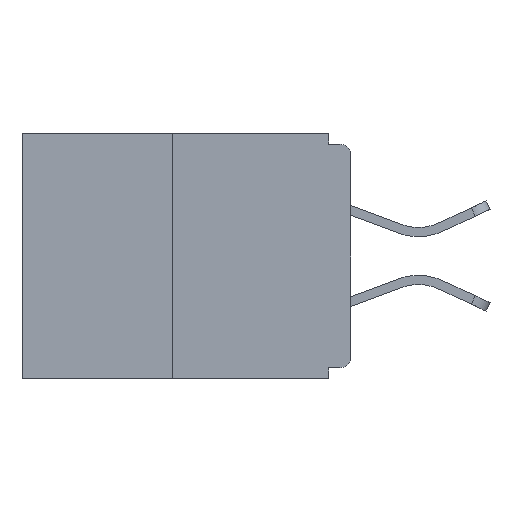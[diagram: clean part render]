
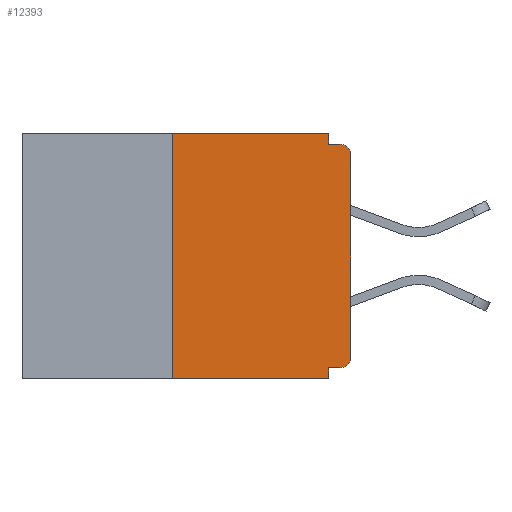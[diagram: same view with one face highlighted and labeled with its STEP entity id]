
A CAD part, left-side view. The second image highlights one B-rep face of the part: STEP entity #12393.
In plain terms, the highlighted planar face has unit normal (-1, 0, 0).
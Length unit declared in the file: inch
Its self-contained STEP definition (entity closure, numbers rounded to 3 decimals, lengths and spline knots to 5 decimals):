
#35 = ORIENTED_EDGE ( 'NONE', *, *, #10973, .T. ) ;
#58 = CARTESIAN_POINT ( 'NONE',  ( 0., 0., -0.03 ) ) ;
#764 = DIRECTION ( 'NONE',  ( 0., 0., -1. ) ) ;
#807 = VECTOR ( 'NONE', #6528, 39.37008 ) ;
#816 = EDGE_CURVE ( 'NONE', #4994, #9443, #3409, .T. ) ;
#1042 = DIRECTION ( 'NONE',  ( 0., 0., -1. ) ) ;
#1137 = CARTESIAN_POINT ( 'NONE',  ( 0., 0.031, -0.328 ) ) ;
#1309 = ORIENTED_EDGE ( 'NONE', *, *, #11805, .F. ) ;
#1310 = ORIENTED_EDGE ( 'NONE', *, *, #8022, .F. ) ;
#1621 = ORIENTED_EDGE ( 'NONE', *, *, #11924, .F. ) ;
#1691 = VERTEX_POINT ( 'NONE', #15045 ) ;
#1877 = ORIENTED_EDGE ( 'NONE', *, *, #17465, .F. ) ;
#2968 = CARTESIAN_POINT ( 'NONE',  ( 0., 0.46, -0.343 ) ) ;
#2973 = EDGE_CURVE ( 'NONE', #4994, #1691, #9009, .T. ) ;
#2989 = ORIENTED_EDGE ( 'NONE', *, *, #15163, .T. ) ;
#3265 = DIRECTION ( 'NONE',  ( 0., -1., 0. ) ) ;
#3409 = LINE ( 'NONE', #2968, #13923 ) ;
#3988 = DIRECTION ( 'NONE',  ( 0., -1., 0. ) ) ;
#4111 = CARTESIAN_POINT ( 'NONE',  ( 0., 0.46, 0. ) ) ;
#4182 = DIRECTION ( 'NONE',  ( 0., 0., -1. ) ) ;
#4279 = VERTEX_POINT ( 'NONE', #58 ) ;
#4339 = CARTESIAN_POINT ( 'NONE',  ( 0., 0., -0.015 ) ) ;
#4845 = ORIENTED_EDGE ( 'NONE', *, *, #12919, .F. ) ;
#4859 = CARTESIAN_POINT ( 'NONE',  ( 0., 0.015, -0.313 ) ) ;
#4976 = CARTESIAN_POINT ( 'NONE',  ( 0., 0.015, -0.015 ) ) ;
#4994 = VERTEX_POINT ( 'NONE', #15820 ) ;
#5221 = CARTESIAN_POINT ( 'NONE',  ( 0., 0.46, 0. ) ) ;
#5409 = CARTESIAN_POINT ( 'NONE',  ( 0., 0.031, -0.343 ) ) ;
#5436 = CIRCLE ( 'NONE', #13734, 0.015 ) ;
#5612 = CARTESIAN_POINT ( 'NONE',  ( 0., 0.015, -0.03 ) ) ;
#5796 = VERTEX_POINT ( 'NONE', #10168 ) ;
#6383 = LINE ( 'NONE', #7894, #13456 ) ;
#6528 = DIRECTION ( 'NONE',  ( 0., 0., 1. ) ) ;
#6610 = DIRECTION ( 'NONE',  ( 0., 0., -1. ) ) ;
#7894 = CARTESIAN_POINT ( 'NONE',  ( 0., 0.031, 0. ) ) ;
#8022 = EDGE_CURVE ( 'NONE', #14456, #11854, #15405, .T. ) ;
#8230 = DIRECTION ( 'NONE',  ( 0., 0., 1. ) ) ;
#8938 = DIRECTION ( 'NONE',  ( -1., 0., 0. ) ) ;
#9009 = LINE ( 'NONE', #9546, #14568 ) ;
#9185 = VECTOR ( 'NONE', #3265, 39.37008 ) ;
#9206 = CARTESIAN_POINT ( 'NONE',  ( 0., 0., -0.328 ) ) ;
#9443 = VERTEX_POINT ( 'NONE', #11286 ) ;
#9546 = CARTESIAN_POINT ( 'NONE',  ( 0., 0.25, 0. ) ) ;
#9635 = CIRCLE ( 'NONE', #11401, 0.015 ) ;
#9689 = LINE ( 'NONE', #4111, #10969 ) ;
#10168 = CARTESIAN_POINT ( 'NONE',  ( 0., 0., -0.313 ) ) ;
#10370 = CARTESIAN_POINT ( 'NONE',  ( 0., 0., 0. ) ) ;
#10440 = ORIENTED_EDGE ( 'NONE', *, *, #14248, .T. ) ;
#10583 = DIRECTION ( 'NONE',  ( 0., 1., 0. ) ) ;
#10796 = LINE ( 'NONE', #5409, #12995 ) ;
#10889 = ORIENTED_EDGE ( 'NONE', *, *, #816, .T. ) ;
#10969 = VECTOR ( 'NONE', #3988, 39.37008 ) ;
#10973 = EDGE_CURVE ( 'NONE', #4279, #11854, #5436, .T. ) ;
#11286 = CARTESIAN_POINT ( 'NONE',  ( 0., 0.031, -0.343 ) ) ;
#11401 = AXIS2_PLACEMENT_3D ( 'NONE', #4859, #8938, #764 ) ;
#11497 = VERTEX_POINT ( 'NONE', #14075 ) ;
#11805 = EDGE_CURVE ( 'NONE', #16619, #13224, #11896, .T. ) ;
#11854 = VERTEX_POINT ( 'NONE', #4976 ) ;
#11896 = LINE ( 'NONE', #9206, #16620 ) ;
#11924 = EDGE_CURVE ( 'NONE', #13224, #9443, #10796, .T. ) ;
#12102 = DIRECTION ( 'NONE',  ( 0., 0., -1. ) ) ;
#12197 = DIRECTION ( 'NONE',  ( 1., 0., 0. ) ) ;
#12393 = ADVANCED_FACE ( 'NONE', ( #14213 ), #17614, .F. ) ;
#12407 = LINE ( 'NONE', #10370, #807 ) ;
#12708 = ORIENTED_EDGE ( 'NONE', *, *, #2973, .F. ) ;
#12767 = DIRECTION ( 'NONE',  ( 0., -1., 0. ) ) ;
#12919 = EDGE_CURVE ( 'NONE', #1691, #11497, #9689, .T. ) ;
#12995 = VECTOR ( 'NONE', #12102, 39.37008 ) ;
#13099 = CARTESIAN_POINT ( 'NONE',  ( 0., 0.015, -0.328 ) ) ;
#13224 = VERTEX_POINT ( 'NONE', #1137 ) ;
#13456 = VECTOR ( 'NONE', #1042, 39.37008 ) ;
#13460 = AXIS2_PLACEMENT_3D ( 'NONE', #5221, #12197, #6610 ) ;
#13734 = AXIS2_PLACEMENT_3D ( 'NONE', #5612, #15278, #4182 ) ;
#13923 = VECTOR ( 'NONE', #12767, 39.37008 ) ;
#14075 = CARTESIAN_POINT ( 'NONE',  ( 0., 0.031, 0. ) ) ;
#14213 = FACE_OUTER_BOUND ( 'NONE', #17084, .T. ) ;
#14248 = EDGE_CURVE ( 'NONE', #16619, #5796, #9635, .T. ) ;
#14456 = VERTEX_POINT ( 'NONE', #16349 ) ;
#14568 = VECTOR ( 'NONE', #8230, 39.37008 ) ;
#15045 = CARTESIAN_POINT ( 'NONE',  ( 0., 0.25, 0. ) ) ;
#15163 = EDGE_CURVE ( 'NONE', #5796, #4279, #12407, .T. ) ;
#15278 = DIRECTION ( 'NONE',  ( -1., 0., 0. ) ) ;
#15405 = LINE ( 'NONE', #4339, #9185 ) ;
#15820 = CARTESIAN_POINT ( 'NONE',  ( 0., 0.25, -0.343 ) ) ;
#16349 = CARTESIAN_POINT ( 'NONE',  ( 0., 0.031, -0.015 ) ) ;
#16619 = VERTEX_POINT ( 'NONE', #13099 ) ;
#16620 = VECTOR ( 'NONE', #10583, 39.37008 ) ;
#17084 = EDGE_LOOP ( 'NONE', ( #4845, #12708, #10889, #1621, #1309, #10440, #2989, #35, #1310, #1877 ) ) ;
#17465 = EDGE_CURVE ( 'NONE', #11497, #14456, #6383, .T. ) ;
#17614 = PLANE ( 'NONE',  #13460 ) ;
